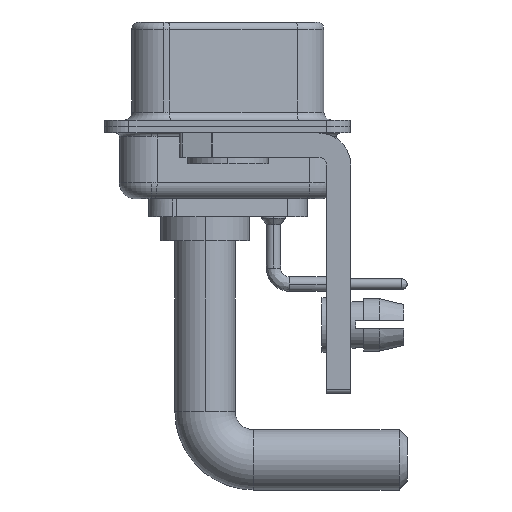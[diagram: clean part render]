
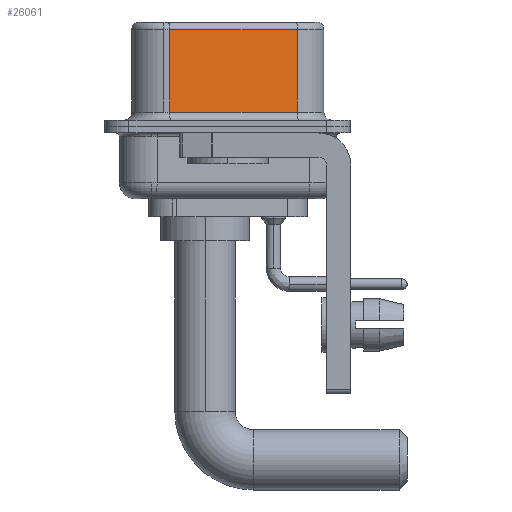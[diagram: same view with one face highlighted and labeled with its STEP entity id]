
A CAD part, left-side view. The second image highlights one B-rep face of the part: STEP entity #26061.
In plain terms, the highlighted planar face has unit normal (-0.985, -0.174, 0).
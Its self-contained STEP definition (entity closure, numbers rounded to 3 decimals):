
#208 = CARTESIAN_POINT ( 'NONE',  ( 5.132, -4.322, 0.9 ) ) ;
#667 = CARTESIAN_POINT ( 'NONE',  ( 5.132, -4.322, 6.02 ) ) ;
#1857 = DIRECTION ( 'NONE',  ( 0., 0., -1. ) ) ;
#2173 = CARTESIAN_POINT ( 'NONE',  ( 5.132, -4.322, 6.02 ) ) ;
#2884 = VERTEX_POINT ( 'NONE', #7535 ) ;
#3036 = VERTEX_POINT ( 'NONE', #208 ) ;
#4254 = DIRECTION ( 'NONE',  ( 0.985, 0.174, 0. ) ) ;
#5454 = ORIENTED_EDGE ( 'NONE', *, *, #19636, .T. ) ;
#6462 = EDGE_CURVE ( 'NONE', #7424, #3036, #24295, .T. ) ;
#7424 = VERTEX_POINT ( 'NONE', #2173 ) ;
#7535 = CARTESIAN_POINT ( 'NONE',  ( 3.73, 3.628, 6.02 ) ) ;
#8329 = CARTESIAN_POINT ( 'NONE',  ( 5.132, -4.322, 0.9 ) ) ;
#8476 = VERTEX_POINT ( 'NONE', #19640 ) ;
#11218 = ORIENTED_EDGE ( 'NONE', *, *, #12871, .T. ) ;
#12334 = DIRECTION ( 'NONE',  ( -0.174, 0.985, 0. ) ) ;
#12367 = VECTOR ( 'NONE', #12569, 1000. ) ;
#12569 = DIRECTION ( 'NONE',  ( 0.174, -0.985, 0. ) ) ;
#12871 = EDGE_CURVE ( 'NONE', #8476, #3036, #16693, .T. ) ;
#14358 = PLANE ( 'NONE',  #18907 ) ;
#14883 = DIRECTION ( 'NONE',  ( -0.174, 0.985, 0. ) ) ;
#15495 = DIRECTION ( 'NONE',  ( 0., 0., -1. ) ) ;
#16444 = VECTOR ( 'NONE', #15495, 1000. ) ;
#16693 = LINE ( 'NONE', #8329, #12367 ) ;
#17472 = LINE ( 'NONE', #25573, #16444 ) ;
#18111 = EDGE_CURVE ( 'NONE', #7424, #2884, #18993, .T. ) ;
#18593 = ORIENTED_EDGE ( 'NONE', *, *, #6462, .F. ) ;
#18907 = AXIS2_PLACEMENT_3D ( 'NONE', #22456, #4254, #12334 ) ;
#18993 = LINE ( 'NONE', #667, #21045 ) ;
#19636 = EDGE_CURVE ( 'NONE', #2884, #8476, #17472, .T. ) ;
#19640 = CARTESIAN_POINT ( 'NONE',  ( 3.73, 3.628, 0.9 ) ) ;
#20435 = CARTESIAN_POINT ( 'NONE',  ( 5.132, -4.322, 6.52 ) ) ;
#20444 = FACE_OUTER_BOUND ( 'NONE', #20543, .T. ) ;
#20543 = EDGE_LOOP ( 'NONE', ( #18593, #25077, #5454, #11218 ) ) ;
#21045 = VECTOR ( 'NONE', #14883, 1000. ) ;
#22456 = CARTESIAN_POINT ( 'NONE',  ( 5.132, -4.322, 6.52 ) ) ;
#24121 = VECTOR ( 'NONE', #1857, 1000. ) ;
#24295 = LINE ( 'NONE', #20435, #24121 ) ;
#25077 = ORIENTED_EDGE ( 'NONE', *, *, #18111, .T. ) ;
#25573 = CARTESIAN_POINT ( 'NONE',  ( 3.73, 3.628, 6.52 ) ) ;
#26061 = ADVANCED_FACE ( 'NONE', ( #20444 ), #14358, .F. ) ;
